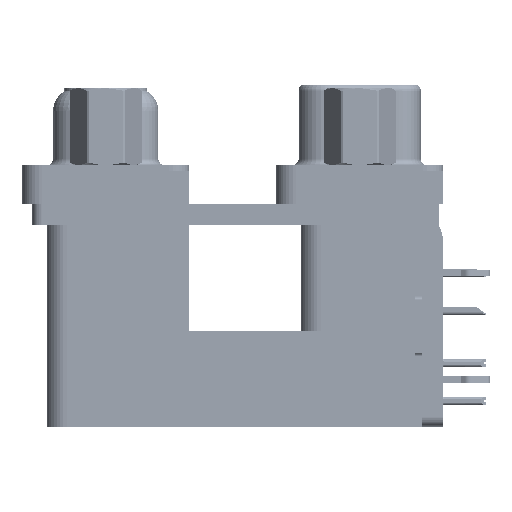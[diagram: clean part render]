
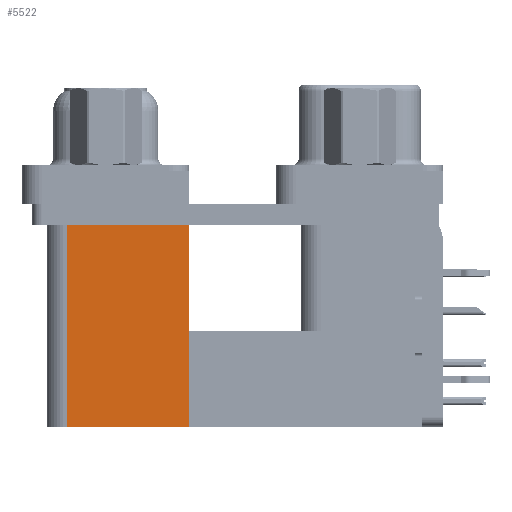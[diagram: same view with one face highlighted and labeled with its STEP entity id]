
A CAD part, left-side view. The second image highlights one B-rep face of the part: STEP entity #5522.
In plain terms, the highlighted planar face has unit normal (-1, 0, 0).
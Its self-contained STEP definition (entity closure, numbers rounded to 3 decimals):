
#4224 = VERTEX_POINT ( 'NONE', #38484 ) ;
#4273 = CARTESIAN_POINT ( 'NONE',  ( 3.7, 21.975, -2.5 ) ) ;
#5375 = ORIENTED_EDGE ( 'NONE', *, *, #61205, .T. ) ;
#5522 = ADVANCED_FACE ( 'NONE', ( #61364 ), #61670, .F. ) ;
#6331 = DIRECTION ( 'NONE',  ( 0., 0., 1. ) ) ;
#7773 = CARTESIAN_POINT ( 'NONE',  ( 3.7, 12.775, -19.2 ) ) ;
#8688 = CARTESIAN_POINT ( 'NONE',  ( 3.7, 12.775, -19.2 ) ) ;
#9358 = DIRECTION ( 'NONE',  ( 0., 1., 0. ) ) ;
#9517 = CARTESIAN_POINT ( 'NONE',  ( 3.7, 21.975, -19.2 ) ) ;
#11143 = VERTEX_POINT ( 'NONE', #4273 ) ;
#15000 = VERTEX_POINT ( 'NONE', #20078 ) ;
#17358 = EDGE_LOOP ( 'NONE', ( #5375, #19746, #26640, #56408 ) ) ;
#18473 = DIRECTION ( 'NONE',  ( 0., 0., -1. ) ) ;
#19746 = ORIENTED_EDGE ( 'NONE', *, *, #44487, .F. ) ;
#20078 = CARTESIAN_POINT ( 'NONE',  ( 3.7, 12.775, -2.5 ) ) ;
#22908 = DIRECTION ( 'NONE',  ( 0., 0., 1. ) ) ;
#23246 = DIRECTION ( 'NONE',  ( 0., 1., 0. ) ) ;
#23808 = DIRECTION ( 'NONE',  ( 1., 0., 0. ) ) ;
#25245 = LINE ( 'NONE', #45133, #31157 ) ;
#26027 = EDGE_CURVE ( 'NONE', #4224, #15000, #56027, .T. ) ;
#26640 = ORIENTED_EDGE ( 'NONE', *, *, #55634, .F. ) ;
#31157 = VECTOR ( 'NONE', #6331, 1000. ) ;
#31669 = VECTOR ( 'NONE', #22908, 1000. ) ;
#33029 = LINE ( 'NONE', #57609, #56909 ) ;
#33339 = LINE ( 'NONE', #48153, #34428 ) ;
#34428 = VECTOR ( 'NONE', #9358, 1000. ) ;
#38484 = CARTESIAN_POINT ( 'NONE',  ( 3.7, 12.775, -19.2 ) ) ;
#44487 = EDGE_CURVE ( 'NONE', #58839, #11143, #25245, .T. ) ;
#45133 = CARTESIAN_POINT ( 'NONE',  ( 3.7, 21.975, -19.2 ) ) ;
#48153 = CARTESIAN_POINT ( 'NONE',  ( 3.7, 12.775, -19.2 ) ) ;
#54061 = AXIS2_PLACEMENT_3D ( 'NONE', #8688, #23808, #18473 ) ;
#55634 = EDGE_CURVE ( 'NONE', #4224, #58839, #33339, .T. ) ;
#56027 = LINE ( 'NONE', #7773, #31669 ) ;
#56408 = ORIENTED_EDGE ( 'NONE', *, *, #26027, .T. ) ;
#56909 = VECTOR ( 'NONE', #23246, 1000. ) ;
#57609 = CARTESIAN_POINT ( 'NONE',  ( 3.7, 12.775, -2.5 ) ) ;
#58839 = VERTEX_POINT ( 'NONE', #9517 ) ;
#61205 = EDGE_CURVE ( 'NONE', #15000, #11143, #33029, .T. ) ;
#61364 = FACE_OUTER_BOUND ( 'NONE', #17358, .T. ) ;
#61670 = PLANE ( 'NONE',  #54061 ) ;
